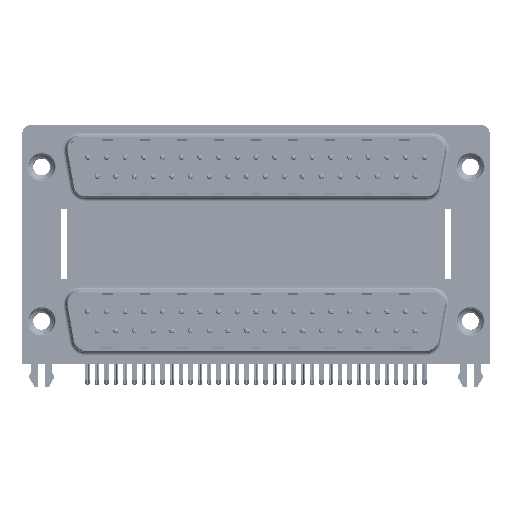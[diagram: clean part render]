
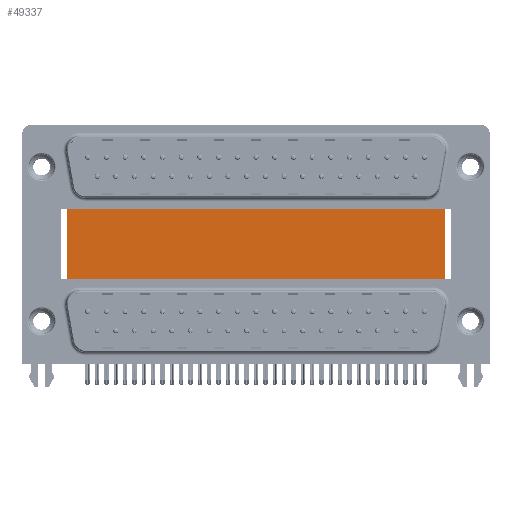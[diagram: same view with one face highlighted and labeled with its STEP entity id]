
A CAD part, top view. The second image highlights one B-rep face of the part: STEP entity #49337.
In plain terms, the highlighted planar face has unit normal (0, 0, 1).
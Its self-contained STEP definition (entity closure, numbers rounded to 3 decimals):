
#3750 = EDGE_CURVE ( 'NONE', #47536, #4542, #43066, .T. ) ;
#4542 = VERTEX_POINT ( 'NONE', #50432 ) ;
#4643 = CARTESIAN_POINT ( 'NONE',  ( 3.79, -3.735, -12. ) ) ;
#6523 = DIRECTION ( 'NONE',  ( 0., -1., 0. ) ) ;
#7047 = ORIENTED_EDGE ( 'NONE', *, *, #41858, .T. ) ;
#7665 = DIRECTION ( 'NONE',  ( 0., -1., 0. ) ) ;
#10845 = CARTESIAN_POINT ( 'NONE',  ( 59.71, 16.585, -12. ) ) ;
#11665 = CARTESIAN_POINT ( 'NONE',  ( 3.79, 16.585, -12. ) ) ;
#15053 = AXIS2_PLACEMENT_3D ( 'NONE', #46253, #35035, #51580 ) ;
#18475 = LINE ( 'NONE', #31287, #35867 ) ;
#18502 = CARTESIAN_POINT ( 'NONE',  ( 59.71, 16.585, -12. ) ) ;
#18726 = PLANE ( 'NONE',  #15053 ) ;
#20716 = EDGE_CURVE ( 'NONE', #30656, #40844, #36765, .T. ) ;
#21561 = EDGE_CURVE ( 'NONE', #30656, #47536, #18475, .T. ) ;
#22194 = ORIENTED_EDGE ( 'NONE', *, *, #21561, .F. ) ;
#23082 = VECTOR ( 'NONE', #6523, 1000. ) ;
#23447 = ORIENTED_EDGE ( 'NONE', *, *, #3750, .F. ) ;
#26204 = ORIENTED_EDGE ( 'NONE', *, *, #20716, .T. ) ;
#26476 = FACE_OUTER_BOUND ( 'NONE', #44260, .T. ) ;
#27061 = CARTESIAN_POINT ( 'NONE',  ( 3.79, 16.585, -12. ) ) ;
#27404 = VECTOR ( 'NONE', #29168, 1000. ) ;
#29168 = DIRECTION ( 'NONE',  ( 1., 0., 0. ) ) ;
#29439 = CARTESIAN_POINT ( 'NONE',  ( 3.79, -3.735, -12. ) ) ;
#30656 = VERTEX_POINT ( 'NONE', #27061 ) ;
#31287 = CARTESIAN_POINT ( 'NONE',  ( 3.79, 16.585, -12. ) ) ;
#33726 = LINE ( 'NONE', #4643, #27404 ) ;
#34077 = VECTOR ( 'NONE', #7665, 1000. ) ;
#35035 = DIRECTION ( 'NONE',  ( 0., 0., -1. ) ) ;
#35867 = VECTOR ( 'NONE', #47570, 1000. ) ;
#36765 = LINE ( 'NONE', #11665, #34077 ) ;
#40844 = VERTEX_POINT ( 'NONE', #29439 ) ;
#41858 = EDGE_CURVE ( 'NONE', #40844, #4542, #33726, .T. ) ;
#43066 = LINE ( 'NONE', #18502, #23082 ) ;
#44260 = EDGE_LOOP ( 'NONE', ( #7047, #23447, #22194, #26204 ) ) ;
#46253 = CARTESIAN_POINT ( 'NONE',  ( 3.79, 16.585, -12. ) ) ;
#47536 = VERTEX_POINT ( 'NONE', #10845 ) ;
#47570 = DIRECTION ( 'NONE',  ( 1., 0., 0. ) ) ;
#49337 = ADVANCED_FACE ( 'NONE', ( #26476 ), #18726, .F. ) ;
#50432 = CARTESIAN_POINT ( 'NONE',  ( 59.71, -3.735, -12. ) ) ;
#51580 = DIRECTION ( 'NONE',  ( -1., 0., 0. ) ) ;
